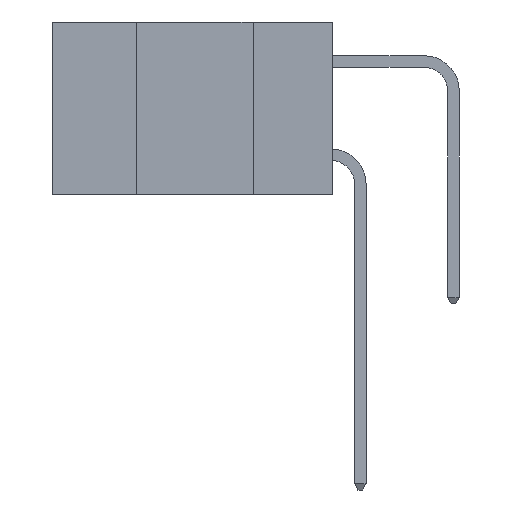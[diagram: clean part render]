
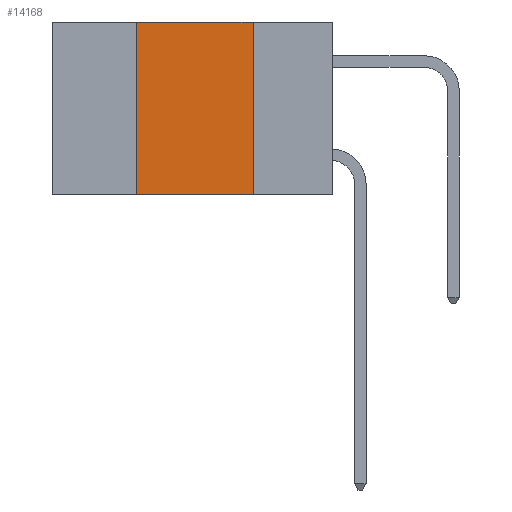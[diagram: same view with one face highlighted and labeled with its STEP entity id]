
A CAD part, left-side view. The second image highlights one B-rep face of the part: STEP entity #14168.
In plain terms, the highlighted planar face has unit normal (-1, 0, 0).
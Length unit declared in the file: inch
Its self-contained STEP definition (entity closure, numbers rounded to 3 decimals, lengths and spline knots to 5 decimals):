
#1468 = CARTESIAN_POINT ( 'NONE',  ( 0., 0.17, 0. ) ) ;
#2015 = CARTESIAN_POINT ( 'NONE',  ( 0., 0.6, 0. ) ) ;
#2837 = LINE ( 'NONE', #2015, #6657 ) ;
#3442 = ORIENTED_EDGE ( 'NONE', *, *, #5971, .F. ) ;
#3555 = VECTOR ( 'NONE', #7509, 39.37008 ) ;
#4530 = VERTEX_POINT ( 'NONE', #1468 ) ;
#4689 = EDGE_LOOP ( 'NONE', ( #19042, #7260, #3442, #15948 ) ) ;
#4859 = EDGE_CURVE ( 'NONE', #8309, #14208, #15322, .T. ) ;
#5971 = EDGE_CURVE ( 'NONE', #8309, #19420, #15679, .T. ) ;
#6657 = VECTOR ( 'NONE', #8557, 39.37008 ) ;
#7046 = EDGE_CURVE ( 'NONE', #19420, #4530, #2837, .T. ) ;
#7260 = ORIENTED_EDGE ( 'NONE', *, *, #7046, .F. ) ;
#7497 = CARTESIAN_POINT ( 'NONE',  ( 0., 0.17, -0.37 ) ) ;
#7509 = DIRECTION ( 'NONE',  ( 0., 0., -1. ) ) ;
#8096 = EDGE_CURVE ( 'NONE', #4530, #14208, #12593, .T. ) ;
#8309 = VERTEX_POINT ( 'NONE', #14176 ) ;
#8557 = DIRECTION ( 'NONE',  ( 0., -1., 0. ) ) ;
#9034 = DIRECTION ( 'NONE',  ( 1., 0., 0. ) ) ;
#9560 = CARTESIAN_POINT ( 'NONE',  ( 0., 0.6, -0.37 ) ) ;
#11733 = VECTOR ( 'NONE', #20000, 39.37008 ) ;
#12179 = CARTESIAN_POINT ( 'NONE',  ( 0., 0.6, 0. ) ) ;
#12593 = LINE ( 'NONE', #19814, #3555 ) ;
#14168 = ADVANCED_FACE ( 'NONE', ( #18538 ), #18196, .F. ) ;
#14176 = CARTESIAN_POINT ( 'NONE',  ( 0., 0.42, -0.37 ) ) ;
#14208 = VERTEX_POINT ( 'NONE', #7497 ) ;
#15322 = LINE ( 'NONE', #9560, #18392 ) ;
#15679 = LINE ( 'NONE', #16926, #11733 ) ;
#15812 = CARTESIAN_POINT ( 'NONE',  ( 0., 0.42, 0. ) ) ;
#15948 = ORIENTED_EDGE ( 'NONE', *, *, #4859, .T. ) ;
#16926 = CARTESIAN_POINT ( 'NONE',  ( 0., 0.42, -0.37 ) ) ;
#17227 = AXIS2_PLACEMENT_3D ( 'NONE', #12179, #9034, #19746 ) ;
#18196 = PLANE ( 'NONE',  #17227 ) ;
#18392 = VECTOR ( 'NONE', #18680, 39.37008 ) ;
#18538 = FACE_OUTER_BOUND ( 'NONE', #4689, .T. ) ;
#18680 = DIRECTION ( 'NONE',  ( 0., -1., 0. ) ) ;
#19042 = ORIENTED_EDGE ( 'NONE', *, *, #8096, .F. ) ;
#19420 = VERTEX_POINT ( 'NONE', #15812 ) ;
#19746 = DIRECTION ( 'NONE',  ( 0., 0., -1. ) ) ;
#19814 = CARTESIAN_POINT ( 'NONE',  ( 0., 0.17, -0.37 ) ) ;
#20000 = DIRECTION ( 'NONE',  ( 0., 0., 1. ) ) ;
